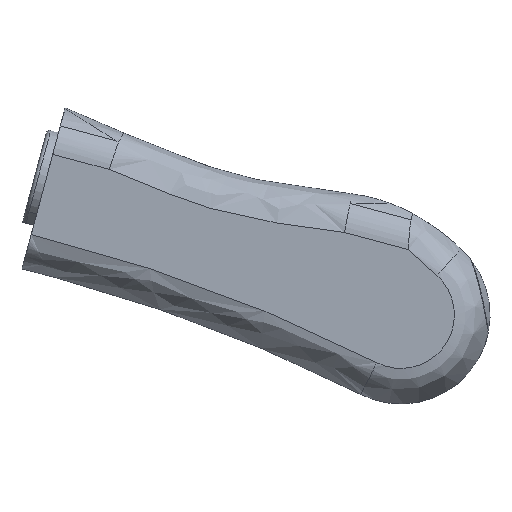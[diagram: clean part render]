
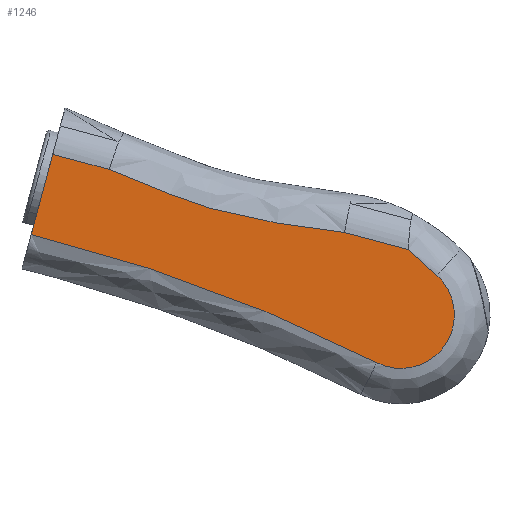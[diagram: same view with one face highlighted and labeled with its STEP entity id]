
A CAD part, left-side view. The second image highlights one B-rep face of the part: STEP entity #1246.
In plain terms, the highlighted planar face has unit normal (-1, 0, 0).
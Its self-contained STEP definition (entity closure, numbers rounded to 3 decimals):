
#77=CIRCLE('',#1350,453.347);
#78=CIRCLE('',#1351,15.);
#150=B_SPLINE_CURVE_WITH_KNOTS('',3,(#3288,#3289,#3290,#3291,#3292,#3293,
#3294,#3295,#3296,#3297),.UNSPECIFIED.,.F.,.F.,(4,1,1,1,1,1,1,4),(-6.862,
-5.923,-4.926,-3.93,-2.933,
-1.937,-0.94,0.),
 .UNSPECIFIED.);
#199=FACE_OUTER_BOUND('',#277,.T.);
#277=EDGE_LOOP('',(#1002,#1003,#1004,#1005,#1006,#1007,#1008));
#332=LINE('',#2042,#412);
#339=LINE('',#2339,#419);
#351=LINE('',#2820,#431);
#352=LINE('',#2954,#432);
#412=VECTOR('',#1458,10.);
#419=VECTOR('',#1479,10.);
#431=VECTOR('',#1503,10.);
#432=VECTOR('',#1506,10.);
#519=VERTEX_POINT('',#2024);
#520=VERTEX_POINT('',#2041);
#540=VERTEX_POINT('',#2325);
#541=VERTEX_POINT('',#2338);
#558=VERTEX_POINT('',#2819);
#562=VERTEX_POINT('',#2941);
#580=VERTEX_POINT('',#3299);
#653=EDGE_CURVE('',#519,#520,#332,.T.);
#677=EDGE_CURVE('',#540,#541,#339,.T.);
#698=EDGE_CURVE('',#541,#558,#351,.T.);
#704=EDGE_CURVE('',#562,#519,#352,.T.);
#735=EDGE_CURVE('',#558,#562,#150,.T.);
#736=EDGE_CURVE('',#540,#580,#77,.T.);
#737=EDGE_CURVE('',#580,#520,#78,.T.);
#1002=ORIENTED_EDGE('',*,*,#704,.F.);
#1003=ORIENTED_EDGE('',*,*,#735,.F.);
#1004=ORIENTED_EDGE('',*,*,#698,.F.);
#1005=ORIENTED_EDGE('',*,*,#677,.F.);
#1006=ORIENTED_EDGE('',*,*,#736,.T.);
#1007=ORIENTED_EDGE('',*,*,#737,.T.);
#1008=ORIENTED_EDGE('',*,*,#653,.F.);
#1194=PLANE('',#1349);
#1246=ADVANCED_FACE('',(#199),#1194,.T.);
#1349=AXIS2_PLACEMENT_3D('',#3298,#1554,#1555);
#1350=AXIS2_PLACEMENT_3D('',#3300,#1556,#1557);
#1351=AXIS2_PLACEMENT_3D('',#3301,#1558,#1559);
#1458=DIRECTION('',(0.,-0.739,-0.674));
#1479=DIRECTION('',(0.,-0.259,0.966));
#1503=DIRECTION('',(0.,-0.966,-0.259));
#1506=DIRECTION('',(0.,-0.966,-0.259));
#1554=DIRECTION('center_axis',(-1.,0.,0.));
#1555=DIRECTION('ref_axis',(0.,-1.,0.));
#1556=DIRECTION('center_axis',(1.,0.,0.));
#1557=DIRECTION('ref_axis',(0.,-0.259,0.966));
#1558=DIRECTION('center_axis',(-1.,0.,0.));
#1559=DIRECTION('ref_axis',(0.,0.452,-0.892));
#2024=CARTESIAN_POINT('',(-17.635,-102.143,-21.657));
#2041=CARTESIAN_POINT('',(-17.635,-110.105,-28.914));
#2042=CARTESIAN_POINT('',(-17.635,-110.105,-28.914));
#2325=CARTESIAN_POINT('',(-17.635,3.816,-17.433));
#2338=CARTESIAN_POINT('',(-17.635,-2.226,5.116));
#2339=CARTESIAN_POINT('',(-17.635,3.789,-17.333));
#2819=CARTESIAN_POINT('',(-17.635,-18.05,0.876));
#2820=CARTESIAN_POINT('',(-17.635,-2.226,5.116));
#2941=CARTESIAN_POINT('',(-17.635,-84.121,-16.828));
#2954=CARTESIAN_POINT('',(-17.635,-2.226,5.116));
#3288=CARTESIAN_POINT('Ctrl Pts',(-17.635,-18.05,0.875));
#3289=CARTESIAN_POINT('Ctrl Pts',(-17.635,-20.932,-0.348));
#3290=CARTESIAN_POINT('Ctrl Pts',(-17.635,-26.895,-2.855));
#3291=CARTESIAN_POINT('Ctrl Pts',(-17.635,-35.994,-6.506));
#3292=CARTESIAN_POINT('Ctrl Pts',(-17.635,-45.4,-9.865));
#3293=CARTESIAN_POINT('Ctrl Pts',(-17.635,-55.057,-12.426));
#3294=CARTESIAN_POINT('Ctrl Pts',(-17.635,-64.886,-14.206));
#3295=CARTESIAN_POINT('Ctrl Pts',(-17.635,-74.593,-15.61));
#3296=CARTESIAN_POINT('Ctrl Pts',(-17.635,-81.01,-16.438));
#3297=CARTESIAN_POINT('Ctrl Pts',(-17.635,-84.121,-16.828));
#3298=CARTESIAN_POINT('Origin',(-17.635,-52.999,-23.417));
#3299=CARTESIAN_POINT('',(-17.635,-93.218,-53.379));
#3300=CARTESIAN_POINT('Origin',(-17.635,111.754,-457.743));
#3301=CARTESIAN_POINT('Origin',(-17.635,-100.,-40.));
